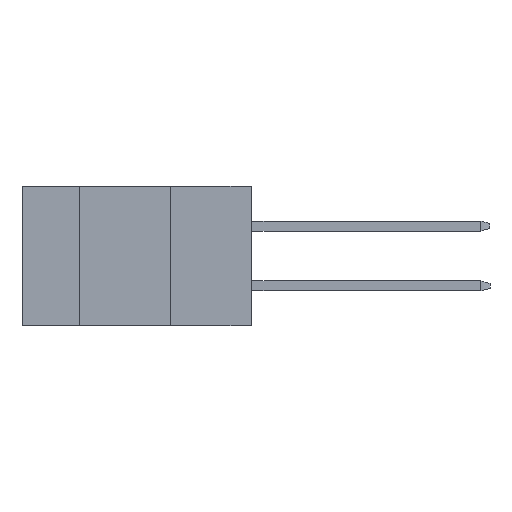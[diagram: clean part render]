
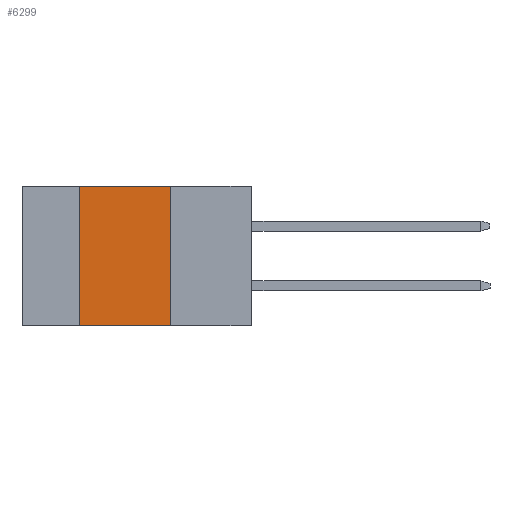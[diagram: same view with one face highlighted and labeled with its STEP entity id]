
A CAD part, left-side view. The second image highlights one B-rep face of the part: STEP entity #6299.
In plain terms, the highlighted planar face has unit normal (-1, 0, 0).
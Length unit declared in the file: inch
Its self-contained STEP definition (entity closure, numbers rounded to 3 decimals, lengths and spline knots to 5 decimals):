
#222 = LINE ( 'NONE', #9199, #18028 ) ;
#319 = CARTESIAN_POINT ( 'NONE',  ( 0., 0.72, -0.437 ) ) ;
#1250 = AXIS2_PLACEMENT_3D ( 'NONE', #16027, #16113, #14649 ) ;
#1306 = EDGE_CURVE ( 'NONE', #6323, #7866, #222, .T. ) ;
#1355 = DIRECTION ( 'NONE',  ( 0., -1., 0. ) ) ;
#1950 = ORIENTED_EDGE ( 'NONE', *, *, #12671, .T. ) ;
#2762 = EDGE_CURVE ( 'NONE', #8348, #6323, #16599, .T. ) ;
#3147 = ORIENTED_EDGE ( 'NONE', *, *, #17232, .F. ) ;
#3837 = ORIENTED_EDGE ( 'NONE', *, *, #1306, .F. ) ;
#4504 = ORIENTED_EDGE ( 'NONE', *, *, #2762, .F. ) ;
#4690 = LINE ( 'NONE', #319, #6377 ) ;
#5919 = CARTESIAN_POINT ( 'NONE',  ( 0., 0.72, 0. ) ) ;
#6299 = ADVANCED_FACE ( 'NONE', ( #11477 ), #10076, .F. ) ;
#6323 = VERTEX_POINT ( 'NONE', #14241 ) ;
#6377 = VECTOR ( 'NONE', #9314, 39.37008 ) ;
#6907 = CARTESIAN_POINT ( 'NONE',  ( 0., 0.54, 0. ) ) ;
#7866 = VERTEX_POINT ( 'NONE', #17182 ) ;
#8229 = CARTESIAN_POINT ( 'NONE',  ( 0., 0.54, -0.437 ) ) ;
#8348 = VERTEX_POINT ( 'NONE', #6907 ) ;
#8919 = CARTESIAN_POINT ( 'NONE',  ( 0., 0.54, -0.437 ) ) ;
#9052 = VECTOR ( 'NONE', #1355, 39.37008 ) ;
#9199 = CARTESIAN_POINT ( 'NONE',  ( 0., 0.254, -0.437 ) ) ;
#9279 = VECTOR ( 'NONE', #14974, 39.37008 ) ;
#9314 = DIRECTION ( 'NONE',  ( 0., -1., 0. ) ) ;
#10076 = PLANE ( 'NONE',  #1250 ) ;
#11477 = FACE_OUTER_BOUND ( 'NONE', #17426, .T. ) ;
#12671 = EDGE_CURVE ( 'NONE', #15475, #7866, #4690, .T. ) ;
#14241 = CARTESIAN_POINT ( 'NONE',  ( 0., 0.254, 0. ) ) ;
#14649 = DIRECTION ( 'NONE',  ( 0., 0., -1. ) ) ;
#14670 = LINE ( 'NONE', #8919, #9279 ) ;
#14861 = DIRECTION ( 'NONE',  ( 0., 0., -1. ) ) ;
#14974 = DIRECTION ( 'NONE',  ( 0., 0., 1. ) ) ;
#15475 = VERTEX_POINT ( 'NONE', #8229 ) ;
#16027 = CARTESIAN_POINT ( 'NONE',  ( 0., 0.72, 0. ) ) ;
#16113 = DIRECTION ( 'NONE',  ( 1., 0., 0. ) ) ;
#16599 = LINE ( 'NONE', #5919, #9052 ) ;
#17182 = CARTESIAN_POINT ( 'NONE',  ( 0., 0.254, -0.437 ) ) ;
#17232 = EDGE_CURVE ( 'NONE', #15475, #8348, #14670, .T. ) ;
#17426 = EDGE_LOOP ( 'NONE', ( #3837, #4504, #3147, #1950 ) ) ;
#18028 = VECTOR ( 'NONE', #14861, 39.37008 ) ;
